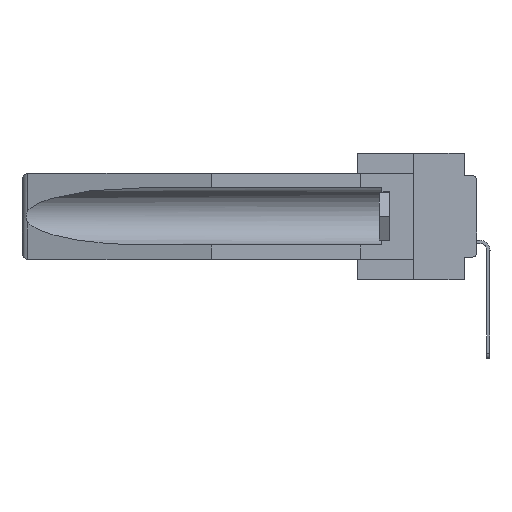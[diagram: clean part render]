
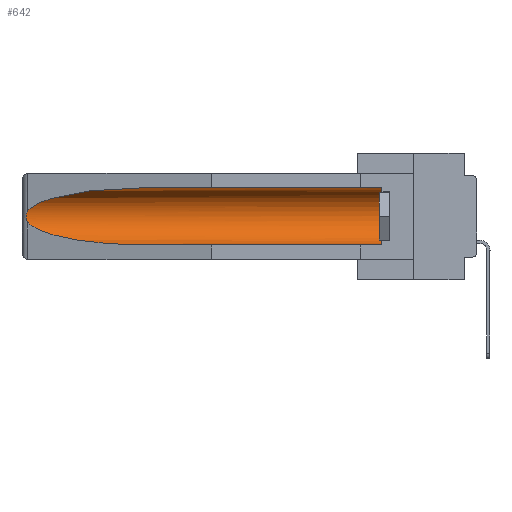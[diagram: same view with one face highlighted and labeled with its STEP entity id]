
A CAD part, left-side view. The second image highlights one B-rep face of the part: STEP entity #642.
In plain terms, the highlighted cylindrical face has radius 2.857 mm (diameter 5.715 mm), a partial arc.
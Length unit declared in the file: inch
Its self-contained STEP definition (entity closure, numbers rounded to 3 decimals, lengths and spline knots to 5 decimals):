
#21 =( BOUNDED_CURVE ( )  B_SPLINE_CURVE ( 3, ( #10967, #16630, #28122, #8182 ),
 .UNSPECIFIED., .F., .F. ) 
 B_SPLINE_CURVE_WITH_KNOTS ( ( 4, 4 ),
 ( 4.71239, 6.08839 ),
 .UNSPECIFIED. ) 
 CURVE ( )  GEOMETRIC_REPRESENTATION_ITEM ( )  RATIONAL_B_SPLINE_CURVE ( ( 1., 0.848, 0.848, 1. ) ) 
 REPRESENTATION_ITEM ( '' )  );
#642 = ADVANCED_FACE ( 'NONE', ( #15498 ), #36146, .F. ) ;
#731 = CARTESIAN_POINT ( 'NONE',  ( 0.26537, 1.52718, -0.19328 ) ) ;
#908 = CARTESIAN_POINT ( 'NONE',  ( 0.26537, 1.52718, -0.19328 ) ) ;
#1114 = VERTEX_POINT ( 'NONE', #7868 ) ;
#1258 = ORIENTED_EDGE ( 'NONE', *, *, #19361, .T. ) ;
#1838 = VECTOR ( 'NONE', #24396, 39.37008 ) ;
#3131 = ORIENTED_EDGE ( 'NONE', *, *, #7300, .T. ) ;
#3217 = AXIS2_PLACEMENT_3D ( 'NONE', #33311, #35635, #10593 ) ;
#3268 = EDGE_CURVE ( 'NONE', #1114, #21404, #21, .T. ) ;
#3353 = B_SPLINE_CURVE_WITH_KNOTS ( 'NONE', 3,
 ( #24774, #22372, #29177, #6808, #28685, #17780, #26332, #4628, #34524, #731 ),
 .UNSPECIFIED., .F., .F.,
 ( 4, 2, 2, 2, 4 ),
 ( 0., 0.00029, 0.00058, 0.00087, 0.00117 ),
 .UNSPECIFIED. ) ;
#4501 = AXIS2_PLACEMENT_3D ( 'NONE', #30870, #14076, #8781 ) ;
#4536 = CARTESIAN_POINT ( 'NONE',  ( 0.155, 0.126, -0.059 ) ) ;
#4628 = CARTESIAN_POINT ( 'NONE',  ( 0.26655, 1.53094, -0.18657 ) ) ;
#4742 = ORIENTED_EDGE ( 'NONE', *, *, #3268, .T. ) ;
#6779 = CARTESIAN_POINT ( 'NONE',  ( 0.26537, 1.52718, -0.19328 ) ) ;
#6808 = CARTESIAN_POINT ( 'NONE',  ( 0.2673, 1.5327, -0.16383 ) ) ;
#7300 = EDGE_CURVE ( 'NONE', #9911, #26399, #35857, .T. ) ;
#7868 = CARTESIAN_POINT ( 'NONE',  ( 0.155, 1.07973, -0.059 ) ) ;
#8011 = CARTESIAN_POINT ( 'NONE',  ( 0.26537, 1.52718, -0.14972 ) ) ;
#8176 = EDGE_CURVE ( 'NONE', #9911, #36163, #32158, .T. ) ;
#8182 = CARTESIAN_POINT ( 'NONE',  ( 0.26537, 1.52718, -0.14972 ) ) ;
#8781 = DIRECTION ( 'NONE',  ( 0., 0., 1. ) ) ;
#9476 = CARTESIAN_POINT ( 'NONE',  ( 0.25451, 1.48313, -0.24835 ) ) ;
#9911 = VERTEX_POINT ( 'NONE', #16621 ) ;
#10593 = DIRECTION ( 'NONE',  ( 0., 0., 1. ) ) ;
#10967 = CARTESIAN_POINT ( 'NONE',  ( 0.155, 1.07973, -0.059 ) ) ;
#11662 = VERTEX_POINT ( 'NONE', #908 ) ;
#14040 = VECTOR ( 'NONE', #27451, 39.37008 ) ;
#14076 = DIRECTION ( 'NONE',  ( 0., -1., 0. ) ) ;
#15498 = FACE_OUTER_BOUND ( 'NONE', #15543, .T. ) ;
#15543 = EDGE_LOOP ( 'NONE', ( #4742, #36205, #1258, #27390, #3131, #30242 ) ) ;
#16621 = CARTESIAN_POINT ( 'NONE',  ( 0.155, 0.126, -0.284 ) ) ;
#16630 = CARTESIAN_POINT ( 'NONE',  ( 0.21114, 1.30732, -0.059 ) ) ;
#17780 = CARTESIAN_POINT ( 'NONE',  ( 0.2675, 1.53308, -0.17534 ) ) ;
#17993 =( BOUNDED_CURVE ( )  B_SPLINE_CURVE ( 3, ( #6779, #9476, #31903, #26371 ),
 .UNSPECIFIED., .F., .F. ) 
 B_SPLINE_CURVE_WITH_KNOTS ( ( 4, 4 ),
 ( 0.1948, 1.5708 ),
 .UNSPECIFIED. ) 
 CURVE ( )  GEOMETRIC_REPRESENTATION_ITEM ( )  RATIONAL_B_SPLINE_CURVE ( ( 1., 0.848, 0.848, 1. ) ) 
 REPRESENTATION_ITEM ( '' )  );
#19361 = EDGE_CURVE ( 'NONE', #11662, #36163, #17993, .T. ) ;
#19967 = EDGE_CURVE ( 'NONE', #21404, #11662, #3353, .T. ) ;
#21404 = VERTEX_POINT ( 'NONE', #8011 ) ;
#21441 = CARTESIAN_POINT ( 'NONE',  ( 0.155, 1.07973, -0.284 ) ) ;
#21975 = CARTESIAN_POINT ( 'NONE',  ( 0.155, -0.30754, -0.284 ) ) ;
#22372 = CARTESIAN_POINT ( 'NONE',  ( 0.26597, 1.52961, -0.15275 ) ) ;
#24396 = DIRECTION ( 'NONE',  ( 0., 1., 0. ) ) ;
#24774 = CARTESIAN_POINT ( 'NONE',  ( 0.26537, 1.52718, -0.14972 ) ) ;
#26332 = CARTESIAN_POINT ( 'NONE',  ( 0.2673, 1.53269, -0.17917 ) ) ;
#26371 = CARTESIAN_POINT ( 'NONE',  ( 0.155, 1.07973, -0.284 ) ) ;
#26399 = VERTEX_POINT ( 'NONE', #4536 ) ;
#27390 = ORIENTED_EDGE ( 'NONE', *, *, #8176, .F. ) ;
#27451 = DIRECTION ( 'NONE',  ( 0., 1., 0. ) ) ;
#28122 = CARTESIAN_POINT ( 'NONE',  ( 0.25451, 1.48313, -0.09465 ) ) ;
#28685 = CARTESIAN_POINT ( 'NONE',  ( 0.2675, 1.53308, -0.16763 ) ) ;
#29177 = CARTESIAN_POINT ( 'NONE',  ( 0.26654, 1.53092, -0.15636 ) ) ;
#29284 = EDGE_CURVE ( 'NONE', #26399, #1114, #30253, .T. ) ;
#30242 = ORIENTED_EDGE ( 'NONE', *, *, #29284, .T. ) ;
#30253 = LINE ( 'NONE', #35951, #14040 ) ;
#30870 = CARTESIAN_POINT ( 'NONE',  ( 0.155, 0.126, -0.1715 ) ) ;
#31903 = CARTESIAN_POINT ( 'NONE',  ( 0.21114, 1.30732, -0.284 ) ) ;
#32158 = LINE ( 'NONE', #21975, #1838 ) ;
#33311 = CARTESIAN_POINT ( 'NONE',  ( 0.155, -0.30754, -0.1715 ) ) ;
#34524 = CARTESIAN_POINT ( 'NONE',  ( 0.26597, 1.5296, -0.19026 ) ) ;
#35635 = DIRECTION ( 'NONE',  ( 0., 1., 0. ) ) ;
#35857 = CIRCLE ( 'NONE', #4501, 0.1125 ) ;
#35951 = CARTESIAN_POINT ( 'NONE',  ( 0.155, -0.30754, -0.059 ) ) ;
#36146 = CYLINDRICAL_SURFACE ( 'NONE', #3217, 0.1125 ) ;
#36163 = VERTEX_POINT ( 'NONE', #21441 ) ;
#36205 = ORIENTED_EDGE ( 'NONE', *, *, #19967, .T. ) ;
